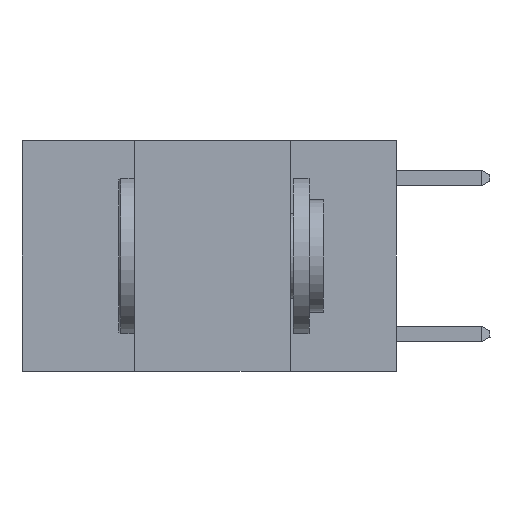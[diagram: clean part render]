
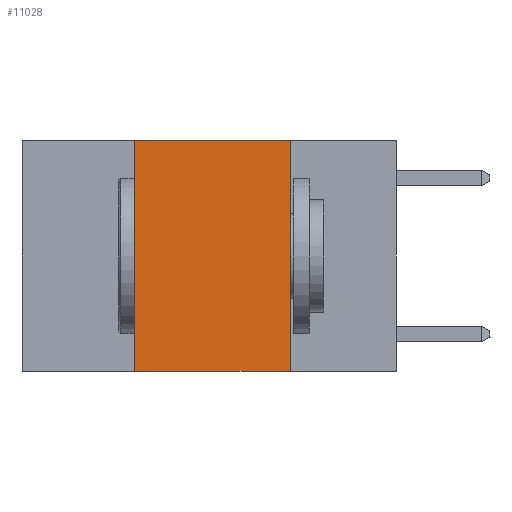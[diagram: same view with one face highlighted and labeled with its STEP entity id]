
A CAD part, left-side view. The second image highlights one B-rep face of the part: STEP entity #11028.
In plain terms, the highlighted planar face has unit normal (-1, 0, 0).
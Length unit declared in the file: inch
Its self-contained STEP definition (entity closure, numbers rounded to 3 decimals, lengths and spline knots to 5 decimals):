
#677 = VECTOR ( 'NONE', #19209, 39.37008 ) ;
#858 = VECTOR ( 'NONE', #9243, 39.37008 ) ;
#913 = LINE ( 'NONE', #10980, #677 ) ;
#964 = VECTOR ( 'NONE', #11097, 39.37008 ) ;
#987 = EDGE_CURVE ( 'NONE', #8427, #4425, #14209, .T. ) ;
#1379 = DIRECTION ( 'NONE',  ( 0., 0., -1. ) ) ;
#1504 = EDGE_LOOP ( 'NONE', ( #2034, #2694, #3738, #14254 ) ) ;
#2034 = ORIENTED_EDGE ( 'NONE', *, *, #987, .F. ) ;
#2694 = ORIENTED_EDGE ( 'NONE', *, *, #12139, .F. ) ;
#3579 = EDGE_CURVE ( 'NONE', #20856, #4425, #16222, .T. ) ;
#3738 = ORIENTED_EDGE ( 'NONE', *, *, #19939, .F. ) ;
#4425 = VERTEX_POINT ( 'NONE', #13491 ) ;
#5826 = CARTESIAN_POINT ( 'NONE',  ( 0., 0.42, 0. ) ) ;
#7082 = VERTEX_POINT ( 'NONE', #5826 ) ;
#7597 = CARTESIAN_POINT ( 'NONE',  ( 0., 0.17, 0. ) ) ;
#8427 = VERTEX_POINT ( 'NONE', #14519 ) ;
#9243 = DIRECTION ( 'NONE',  ( 0., 0., 1. ) ) ;
#10701 = PLANE ( 'NONE',  #14850 ) ;
#10980 = CARTESIAN_POINT ( 'NONE',  ( 0., 0.6, 0. ) ) ;
#11028 = ADVANCED_FACE ( 'NONE', ( #14296 ), #10701, .F. ) ;
#11097 = DIRECTION ( 'NONE',  ( 0., -1., 0. ) ) ;
#11902 = LINE ( 'NONE', #14378, #858 ) ;
#12139 = EDGE_CURVE ( 'NONE', #7082, #8427, #913, .T. ) ;
#12445 = DIRECTION ( 'NONE',  ( 1., 0., 0. ) ) ;
#13491 = CARTESIAN_POINT ( 'NONE',  ( 0., 0.17, -0.37 ) ) ;
#13650 = VECTOR ( 'NONE', #21083, 39.37008 ) ;
#14018 = CARTESIAN_POINT ( 'NONE',  ( 0., 0.6, 0. ) ) ;
#14209 = LINE ( 'NONE', #7597, #13650 ) ;
#14254 = ORIENTED_EDGE ( 'NONE', *, *, #3579, .T. ) ;
#14296 = FACE_OUTER_BOUND ( 'NONE', #1504, .T. ) ;
#14378 = CARTESIAN_POINT ( 'NONE',  ( 0., 0.42, 0. ) ) ;
#14519 = CARTESIAN_POINT ( 'NONE',  ( 0., 0.17, 0. ) ) ;
#14850 = AXIS2_PLACEMENT_3D ( 'NONE', #14018, #12445, #1379 ) ;
#14855 = CARTESIAN_POINT ( 'NONE',  ( 0., 0.42, -0.37 ) ) ;
#16141 = CARTESIAN_POINT ( 'NONE',  ( 0., 0.6, -0.37 ) ) ;
#16222 = LINE ( 'NONE', #16141, #964 ) ;
#19209 = DIRECTION ( 'NONE',  ( 0., -1., 0. ) ) ;
#19939 = EDGE_CURVE ( 'NONE', #20856, #7082, #11902, .T. ) ;
#20856 = VERTEX_POINT ( 'NONE', #14855 ) ;
#21083 = DIRECTION ( 'NONE',  ( 0., 0., -1. ) ) ;
